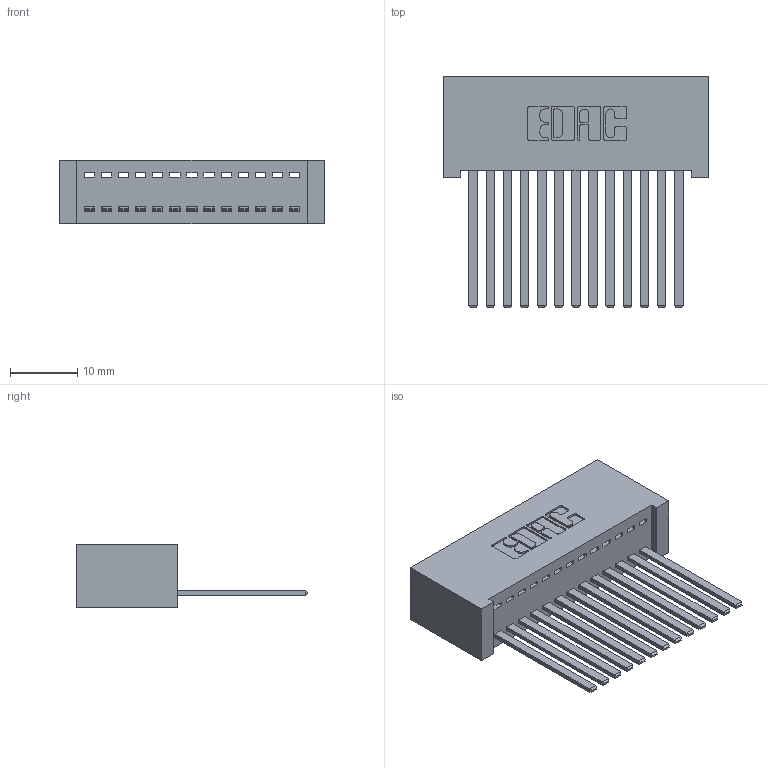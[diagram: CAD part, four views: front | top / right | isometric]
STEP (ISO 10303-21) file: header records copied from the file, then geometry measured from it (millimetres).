
FILE_DESCRIPTION (( 'STEP AP203' ), '1' );
FILE_NAME ('392-013-544-101.STEP', '2019-10-07T01:57:29', ( '' ), ( '' ), 'SwSTEP 2.0', 'SolidWorks 2016', '' );
FILE_SCHEMA (( 'CONFIG_CONTROL_DESIGN' ));
Length unit declared in the file: inch
Products named in the file (3): 345-292-001_345-293-144; 392-013-544-101; 342 Part_Lugless
Assembly tree (14 placements, depth 2):
  392-013-544-101
    342 Part_Lugless
    345-292-001_345-293-144  x13
Bounding box: 39.27 x 34.3 x 9.4 mm (x, y, z)
Volume: 3895.8 mm3; surface area: 5931.1 mm2
Topology: 14 solids, 14 shells, 778 faces, 2329 edges, 1534 vertices
Faces by surface type: plane 556, cylinder 222
Entity records: 11105 total; most frequent: CARTESIAN_POINT 1925, ORIENTED_EDGE 1874, DIRECTION 1671, EDGE_CURVE 937, VECTOR 821, LINE 821, VERTEX_POINT 622, AXIS2_PLACEMENT_3D 425
